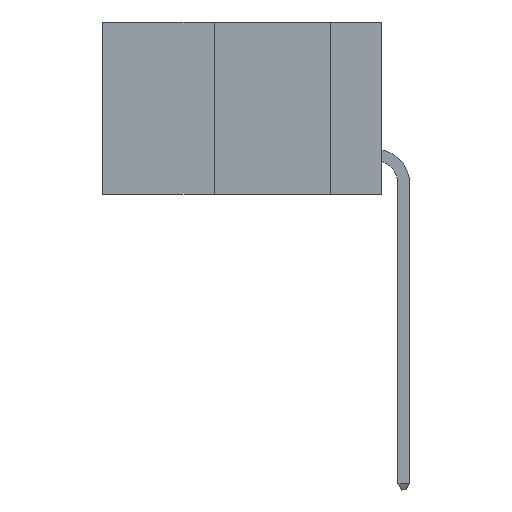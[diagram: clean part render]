
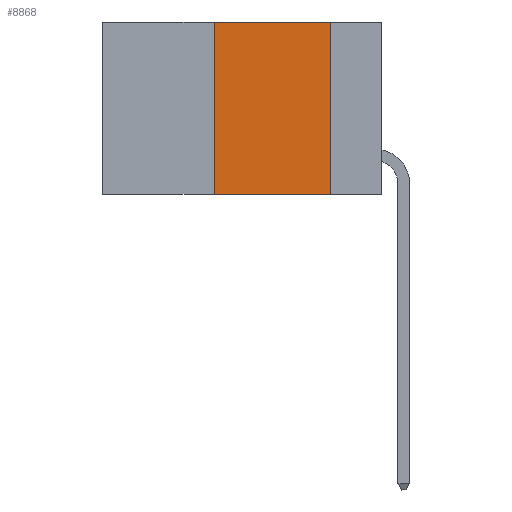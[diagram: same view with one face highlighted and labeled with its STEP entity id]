
A CAD part, left-side view. The second image highlights one B-rep face of the part: STEP entity #8868.
In plain terms, the highlighted planar face has unit normal (-1, 0, 0).
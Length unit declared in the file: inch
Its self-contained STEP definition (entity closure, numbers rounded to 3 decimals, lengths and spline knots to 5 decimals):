
#3 = EDGE_CURVE ( 'NONE', #11536, #4006, #9134, .T. ) ;
#90 = DIRECTION ( 'NONE',  ( 0., 0., 1. ) ) ;
#314 = CARTESIAN_POINT ( 'NONE',  ( 0., 0.36, -0.37 ) ) ;
#908 = LINE ( 'NONE', #18812, #15120 ) ;
#1429 = DIRECTION ( 'NONE',  ( 0., 0., -1. ) ) ;
#1514 = DIRECTION ( 'NONE',  ( 0., -1., 0. ) ) ;
#2442 = EDGE_CURVE ( 'NONE', #19597, #10505, #5570, .T. ) ;
#2671 = VECTOR ( 'NONE', #1429, 39.37008 ) ;
#2969 = CARTESIAN_POINT ( 'NONE',  ( 0., 0.11, -0.37 ) ) ;
#3337 = CARTESIAN_POINT ( 'NONE',  ( 0., 0.36, 0. ) ) ;
#3689 = ORIENTED_EDGE ( 'NONE', *, *, #2442, .F. ) ;
#4006 = VERTEX_POINT ( 'NONE', #2969 ) ;
#4255 = DIRECTION ( 'NONE',  ( 1., 0., 0. ) ) ;
#4295 = VECTOR ( 'NONE', #90, 39.37008 ) ;
#4615 = EDGE_CURVE ( 'NONE', #19597, #4006, #13194, .T. ) ;
#4791 = AXIS2_PLACEMENT_3D ( 'NONE', #14136, #4255, #20766 ) ;
#5570 = LINE ( 'NONE', #3337, #4295 ) ;
#5583 = DIRECTION ( 'NONE',  ( 0., -1., 0. ) ) ;
#6851 = CARTESIAN_POINT ( 'NONE',  ( 0., 0.11, 0. ) ) ;
#6974 = ORIENTED_EDGE ( 'NONE', *, *, #3, .F. ) ;
#8280 = EDGE_LOOP ( 'NONE', ( #6974, #15476, #3689, #16497 ) ) ;
#8868 = ADVANCED_FACE ( 'NONE', ( #10742 ), #17592, .F. ) ;
#9134 = LINE ( 'NONE', #14859, #2671 ) ;
#10505 = VERTEX_POINT ( 'NONE', #16988 ) ;
#10742 = FACE_OUTER_BOUND ( 'NONE', #8280, .T. ) ;
#11536 = VERTEX_POINT ( 'NONE', #6851 ) ;
#13194 = LINE ( 'NONE', #14733, #14502 ) ;
#14136 = CARTESIAN_POINT ( 'NONE',  ( 0., 0.6, 0. ) ) ;
#14502 = VECTOR ( 'NONE', #1514, 39.37008 ) ;
#14733 = CARTESIAN_POINT ( 'NONE',  ( 0., 0.6, -0.37 ) ) ;
#14859 = CARTESIAN_POINT ( 'NONE',  ( 0., 0.11, 0. ) ) ;
#15120 = VECTOR ( 'NONE', #5583, 39.37008 ) ;
#15476 = ORIENTED_EDGE ( 'NONE', *, *, #15930, .F. ) ;
#15930 = EDGE_CURVE ( 'NONE', #10505, #11536, #908, .T. ) ;
#16497 = ORIENTED_EDGE ( 'NONE', *, *, #4615, .T. ) ;
#16988 = CARTESIAN_POINT ( 'NONE',  ( 0., 0.36, 0. ) ) ;
#17592 = PLANE ( 'NONE',  #4791 ) ;
#18812 = CARTESIAN_POINT ( 'NONE',  ( 0., 0.6, 0. ) ) ;
#19597 = VERTEX_POINT ( 'NONE', #314 ) ;
#20766 = DIRECTION ( 'NONE',  ( 0., 0., -1. ) ) ;
